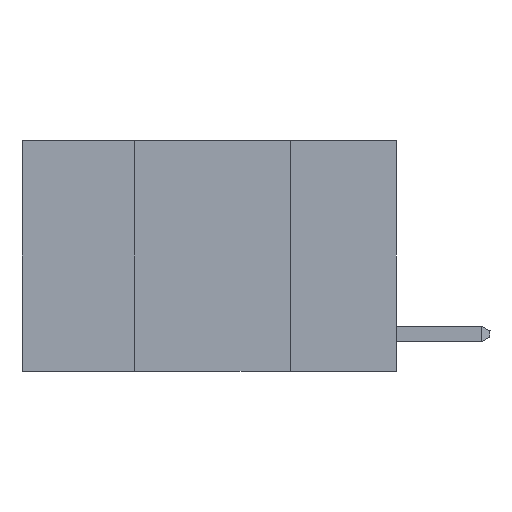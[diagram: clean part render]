
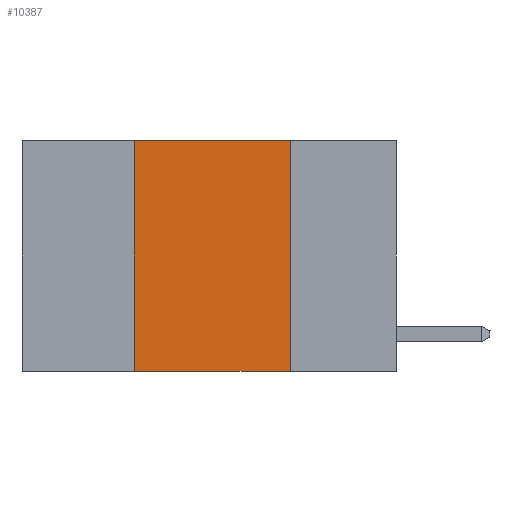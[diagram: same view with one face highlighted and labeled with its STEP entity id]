
A CAD part, left-side view. The second image highlights one B-rep face of the part: STEP entity #10387.
In plain terms, the highlighted planar face has unit normal (-1, 0, 0).
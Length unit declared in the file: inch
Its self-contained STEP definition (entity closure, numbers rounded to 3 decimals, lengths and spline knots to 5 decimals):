
#527 = CARTESIAN_POINT ( 'NONE',  ( 0., 0.17, -0.37 ) ) ;
#1285 = CARTESIAN_POINT ( 'NONE',  ( 0., 0.6, 0. ) ) ;
#2034 = VERTEX_POINT ( 'NONE', #3139 ) ;
#2370 = ORIENTED_EDGE ( 'NONE', *, *, #15284, .F. ) ;
#2388 = FACE_OUTER_BOUND ( 'NONE', #14833, .T. ) ;
#3139 = CARTESIAN_POINT ( 'NONE',  ( 0., 0.17, 0. ) ) ;
#5000 = DIRECTION ( 'NONE',  ( 0., 0., 1. ) ) ;
#5411 = DIRECTION ( 'NONE',  ( 0., 0., -1. ) ) ;
#5664 = CARTESIAN_POINT ( 'NONE',  ( 0., 0.6, -0.37 ) ) ;
#6027 = EDGE_CURVE ( 'NONE', #2034, #10315, #18212, .T. ) ;
#6795 = DIRECTION ( 'NONE',  ( 0., -1., 0. ) ) ;
#7035 = VECTOR ( 'NONE', #18497, 39.37008 ) ;
#8118 = PLANE ( 'NONE',  #15412 ) ;
#8591 = CARTESIAN_POINT ( 'NONE',  ( 0., 0.42, 0. ) ) ;
#9989 = VERTEX_POINT ( 'NONE', #17835 ) ;
#10315 = VERTEX_POINT ( 'NONE', #527 ) ;
#10387 = ADVANCED_FACE ( 'NONE', ( #2388 ), #8118, .F. ) ;
#11730 = DIRECTION ( 'NONE',  ( 0., 0., -1. ) ) ;
#12080 = LINE ( 'NONE', #8591, #16441 ) ;
#13230 = VECTOR ( 'NONE', #5411, 39.37008 ) ;
#14255 = VERTEX_POINT ( 'NONE', #16834 ) ;
#14833 = EDGE_LOOP ( 'NONE', ( #19544, #2370, #22443, #23611 ) ) ;
#15284 = EDGE_CURVE ( 'NONE', #9989, #2034, #18604, .T. ) ;
#15412 = AXIS2_PLACEMENT_3D ( 'NONE', #20945, #22810, #11730 ) ;
#15610 = LINE ( 'NONE', #5664, #7035 ) ;
#16441 = VECTOR ( 'NONE', #5000, 39.37008 ) ;
#16834 = CARTESIAN_POINT ( 'NONE',  ( 0., 0.42, -0.37 ) ) ;
#17835 = CARTESIAN_POINT ( 'NONE',  ( 0., 0.42, 0. ) ) ;
#18028 = VECTOR ( 'NONE', #6795, 39.37008 ) ;
#18212 = LINE ( 'NONE', #23723, #13230 ) ;
#18497 = DIRECTION ( 'NONE',  ( 0., -1., 0. ) ) ;
#18604 = LINE ( 'NONE', #1285, #18028 ) ;
#19544 = ORIENTED_EDGE ( 'NONE', *, *, #6027, .F. ) ;
#20945 = CARTESIAN_POINT ( 'NONE',  ( 0., 0.6, 0. ) ) ;
#21255 = EDGE_CURVE ( 'NONE', #14255, #10315, #15610, .T. ) ;
#22443 = ORIENTED_EDGE ( 'NONE', *, *, #22488, .F. ) ;
#22488 = EDGE_CURVE ( 'NONE', #14255, #9989, #12080, .T. ) ;
#22810 = DIRECTION ( 'NONE',  ( 1., 0., 0. ) ) ;
#23611 = ORIENTED_EDGE ( 'NONE', *, *, #21255, .T. ) ;
#23723 = CARTESIAN_POINT ( 'NONE',  ( 0., 0.17, 0. ) ) ;
